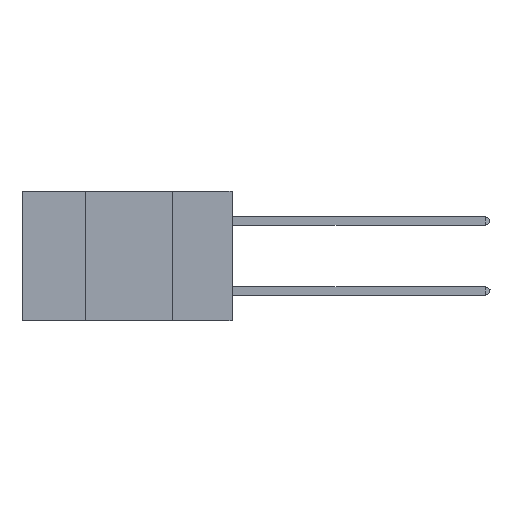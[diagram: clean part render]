
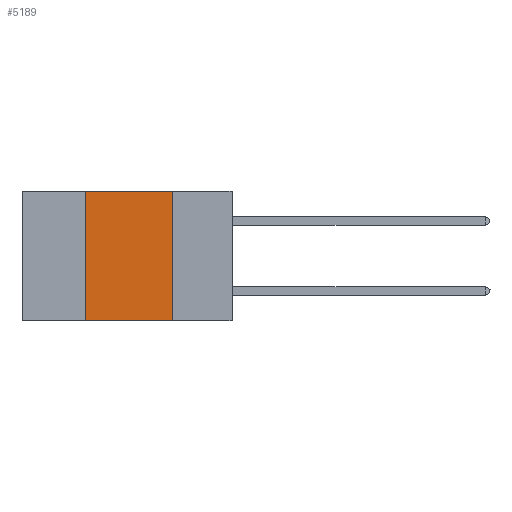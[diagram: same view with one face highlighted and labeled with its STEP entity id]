
A CAD part, left-side view. The second image highlights one B-rep face of the part: STEP entity #5189.
In plain terms, the highlighted planar face has unit normal (-1, 0, 0).
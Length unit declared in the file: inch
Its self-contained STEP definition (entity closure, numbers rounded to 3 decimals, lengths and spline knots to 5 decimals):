
#53 = DIRECTION ( 'NONE',  ( 1., 0., 0. ) ) ;
#190 = PLANE ( 'NONE',  #755 ) ;
#281 = CARTESIAN_POINT ( 'NONE',  ( 0., 0.6, 0. ) ) ;
#297 = EDGE_LOOP ( 'NONE', ( #12163, #21706, #15326, #4855 ) ) ;
#450 = LINE ( 'NONE', #17556, #8818 ) ;
#755 = AXIS2_PLACEMENT_3D ( 'NONE', #23697, #53, #23432 ) ;
#1642 = DIRECTION ( 'NONE',  ( 0., 0., -1. ) ) ;
#3112 = EDGE_CURVE ( 'NONE', #19984, #8488, #10259, .T. ) ;
#4422 = VECTOR ( 'NONE', #27004, 39.37008 ) ;
#4855 = ORIENTED_EDGE ( 'NONE', *, *, #21836, .T. ) ;
#5189 = ADVANCED_FACE ( 'NONE', ( #21903 ), #190, .F. ) ;
#5985 = CARTESIAN_POINT ( 'NONE',  ( 0., 0.42, 0. ) ) ;
#6721 = DIRECTION ( 'NONE',  ( 0., -1., 0. ) ) ;
#7855 = CARTESIAN_POINT ( 'NONE',  ( 0., 0.17, 0. ) ) ;
#8184 = CARTESIAN_POINT ( 'NONE',  ( 0., 0.17, -0.37 ) ) ;
#8191 = LINE ( 'NONE', #5985, #4422 ) ;
#8488 = VERTEX_POINT ( 'NONE', #8184 ) ;
#8818 = VECTOR ( 'NONE', #6721, 39.37008 ) ;
#9622 = EDGE_CURVE ( 'NONE', #17869, #21248, #8191, .T. ) ;
#10259 = LINE ( 'NONE', #16636, #19608 ) ;
#12163 = ORIENTED_EDGE ( 'NONE', *, *, #3112, .F. ) ;
#12229 = VECTOR ( 'NONE', #25882, 39.37008 ) ;
#12933 = LINE ( 'NONE', #281, #12229 ) ;
#15326 = ORIENTED_EDGE ( 'NONE', *, *, #9622, .F. ) ;
#16636 = CARTESIAN_POINT ( 'NONE',  ( 0., 0.17, 0. ) ) ;
#17556 = CARTESIAN_POINT ( 'NONE',  ( 0., 0.6, -0.37 ) ) ;
#17666 = CARTESIAN_POINT ( 'NONE',  ( 0., 0.42, 0. ) ) ;
#17869 = VERTEX_POINT ( 'NONE', #23671 ) ;
#18317 = EDGE_CURVE ( 'NONE', #21248, #19984, #12933, .T. ) ;
#19608 = VECTOR ( 'NONE', #1642, 39.37008 ) ;
#19984 = VERTEX_POINT ( 'NONE', #7855 ) ;
#21248 = VERTEX_POINT ( 'NONE', #17666 ) ;
#21706 = ORIENTED_EDGE ( 'NONE', *, *, #18317, .F. ) ;
#21836 = EDGE_CURVE ( 'NONE', #17869, #8488, #450, .T. ) ;
#21903 = FACE_OUTER_BOUND ( 'NONE', #297, .T. ) ;
#23432 = DIRECTION ( 'NONE',  ( 0., 0., -1. ) ) ;
#23671 = CARTESIAN_POINT ( 'NONE',  ( 0., 0.42, -0.37 ) ) ;
#23697 = CARTESIAN_POINT ( 'NONE',  ( 0., 0.6, 0. ) ) ;
#25882 = DIRECTION ( 'NONE',  ( 0., -1., 0. ) ) ;
#27004 = DIRECTION ( 'NONE',  ( 0., 0., 1. ) ) ;
